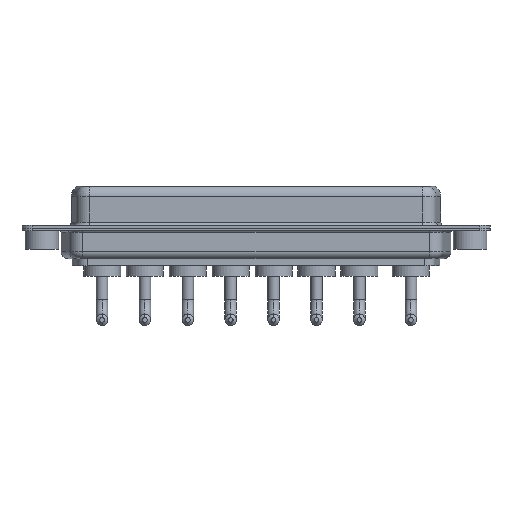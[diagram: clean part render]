
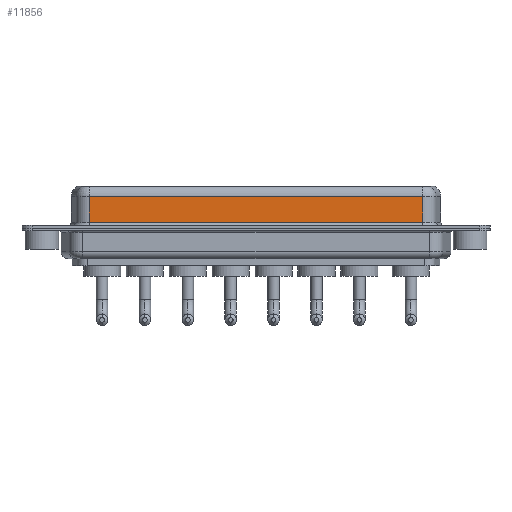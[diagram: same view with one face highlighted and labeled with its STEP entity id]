
A CAD part, front view. The second image highlights one B-rep face of the part: STEP entity #11856.
In plain terms, the highlighted planar face has unit normal (0, -1, 0).
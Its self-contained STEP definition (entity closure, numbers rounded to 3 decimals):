
#533 = ORIENTED_EDGE ( 'NONE', *, *, #7318, .T. ) ;
#713 = ORIENTED_EDGE ( 'NONE', *, *, #4423, .F. ) ;
#1177 = CARTESIAN_POINT ( 'NONE',  ( 56.462, -3.95, 6.4 ) ) ;
#2608 = VERTEX_POINT ( 'NONE', #3459 ) ;
#3133 = VERTEX_POINT ( 'NONE', #7817 ) ;
#3217 = LINE ( 'NONE', #7139, #11094 ) ;
#3279 = EDGE_LOOP ( 'NONE', ( #713, #9444, #6509, #533 ) ) ;
#3371 = VECTOR ( 'NONE', #3642, 1000. ) ;
#3459 = CARTESIAN_POINT ( 'NONE',  ( 7.038, -3.95, 4.65 ) ) ;
#3642 = DIRECTION ( 'NONE',  ( 0., 0., -1. ) ) ;
#3961 = AXIS2_PLACEMENT_3D ( 'NONE', #1177, #6355, #12319 ) ;
#4423 = EDGE_CURVE ( 'NONE', #10726, #6530, #6552, .T. ) ;
#5125 = CARTESIAN_POINT ( 'NONE',  ( 56.462, -3.95, 0.9 ) ) ;
#5155 = PLANE ( 'NONE',  #3961 ) ;
#5860 = CARTESIAN_POINT ( 'NONE',  ( 56.462, -3.95, 4.65 ) ) ;
#5886 = LINE ( 'NONE', #10047, #12455 ) ;
#6129 = DIRECTION ( 'NONE',  ( 0., 0., -1. ) ) ;
#6355 = DIRECTION ( 'NONE',  ( 0., 1., 0. ) ) ;
#6509 = ORIENTED_EDGE ( 'NONE', *, *, #13144, .T. ) ;
#6530 = VERTEX_POINT ( 'NONE', #5125 ) ;
#6552 = LINE ( 'NONE', #12859, #3371 ) ;
#7139 = CARTESIAN_POINT ( 'NONE',  ( 56.462, -3.95, 4.65 ) ) ;
#7216 = VECTOR ( 'NONE', #6129, 1000. ) ;
#7318 = EDGE_CURVE ( 'NONE', #3133, #6530, #5886, .T. ) ;
#7817 = CARTESIAN_POINT ( 'NONE',  ( 7.038, -3.95, 0.9 ) ) ;
#8024 = DIRECTION ( 'NONE',  ( 1., 0., 0. ) ) ;
#9444 = ORIENTED_EDGE ( 'NONE', *, *, #13012, .T. ) ;
#10047 = CARTESIAN_POINT ( 'NONE',  ( 56.462, -3.95, 0.9 ) ) ;
#10321 = FACE_OUTER_BOUND ( 'NONE', #3279, .T. ) ;
#10726 = VERTEX_POINT ( 'NONE', #5860 ) ;
#11094 = VECTOR ( 'NONE', #13236, 1000. ) ;
#11444 = CARTESIAN_POINT ( 'NONE',  ( 7.038, -3.95, 6.4 ) ) ;
#11856 = ADVANCED_FACE ( 'NONE', ( #10321 ), #5155, .F. ) ;
#12319 = DIRECTION ( 'NONE',  ( 0., 0., 1. ) ) ;
#12455 = VECTOR ( 'NONE', #8024, 1000. ) ;
#12859 = CARTESIAN_POINT ( 'NONE',  ( 56.462, -3.95, 6.4 ) ) ;
#13012 = EDGE_CURVE ( 'NONE', #10726, #2608, #3217, .T. ) ;
#13144 = EDGE_CURVE ( 'NONE', #2608, #3133, #13164, .T. ) ;
#13164 = LINE ( 'NONE', #11444, #7216 ) ;
#13236 = DIRECTION ( 'NONE',  ( -1., 0., 0. ) ) ;
